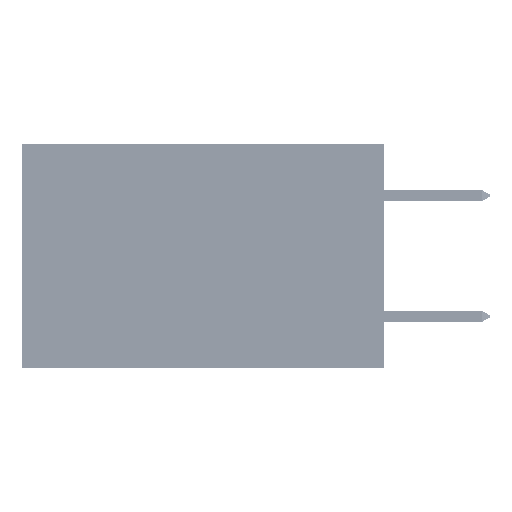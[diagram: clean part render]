
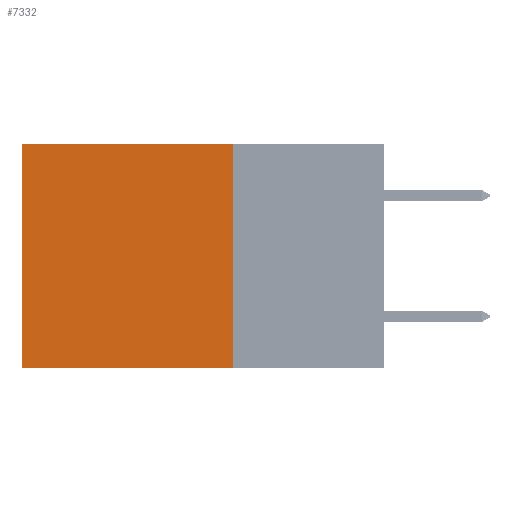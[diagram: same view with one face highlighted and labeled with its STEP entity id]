
A CAD part, left-side view. The second image highlights one B-rep face of the part: STEP entity #7332.
In plain terms, the highlighted planar face has unit normal (-1, 0, 0).
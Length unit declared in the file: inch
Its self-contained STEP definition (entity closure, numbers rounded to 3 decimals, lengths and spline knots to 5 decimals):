
#388 = CARTESIAN_POINT ( 'NONE',  ( 0.2875, 0.6, 0. ) ) ;
#1718 = DIRECTION ( 'NONE',  ( 0., 1., 0. ) ) ;
#2226 = DIRECTION ( 'NONE',  ( 1., 0., 0. ) ) ;
#3516 = AXIS2_PLACEMENT_3D ( 'NONE', #24717, #2226, #6004 ) ;
#3786 = VECTOR ( 'NONE', #7145, 39.37008 ) ;
#4323 = EDGE_LOOP ( 'NONE', ( #27714, #42991, #12882, #36826 ) ) ;
#5016 = EDGE_CURVE ( 'NONE', #23131, #36613, #47746, .T. ) ;
#6004 = DIRECTION ( 'NONE',  ( 0., 0., -1. ) ) ;
#6733 = CARTESIAN_POINT ( 'NONE',  ( 0.2875, 0.25, 0. ) ) ;
#7145 = DIRECTION ( 'NONE',  ( 0., 1., 0. ) ) ;
#7332 = ADVANCED_FACE ( 'NONE', ( #18770 ), #43321, .F. ) ;
#7511 = CARTESIAN_POINT ( 'NONE',  ( 0.2875, 0.6, 0. ) ) ;
#11528 = DIRECTION ( 'NONE',  ( 0., 0., -1. ) ) ;
#12882 = ORIENTED_EDGE ( 'NONE', *, *, #30175, .F. ) ;
#14334 = CARTESIAN_POINT ( 'NONE',  ( 0.2875, 0.6, -0.37 ) ) ;
#18770 = FACE_OUTER_BOUND ( 'NONE', #4323, .T. ) ;
#19137 = DIRECTION ( 'NONE',  ( 0., 0., -1. ) ) ;
#19555 = VERTEX_POINT ( 'NONE', #6733 ) ;
#21462 = VECTOR ( 'NONE', #11528, 39.37008 ) ;
#22094 = CARTESIAN_POINT ( 'NONE',  ( 0.2875, 0.25, 0. ) ) ;
#23131 = VERTEX_POINT ( 'NONE', #388 ) ;
#24717 = CARTESIAN_POINT ( 'NONE',  ( 0.2875, 0.25, 0. ) ) ;
#25836 = CARTESIAN_POINT ( 'NONE',  ( 0.2875, 0.25, -0.37 ) ) ;
#25905 = LINE ( 'NONE', #27673, #41194 ) ;
#27673 = CARTESIAN_POINT ( 'NONE',  ( 0.2875, 0.25, 0. ) ) ;
#27714 = ORIENTED_EDGE ( 'NONE', *, *, #5016, .T. ) ;
#27750 = EDGE_CURVE ( 'NONE', #19555, #23131, #25905, .T. ) ;
#28917 = VECTOR ( 'NONE', #19137, 39.37008 ) ;
#30101 = EDGE_CURVE ( 'NONE', #39556, #36613, #32620, .T. ) ;
#30175 = EDGE_CURVE ( 'NONE', #19555, #39556, #36176, .T. ) ;
#32620 = LINE ( 'NONE', #25836, #3786 ) ;
#36176 = LINE ( 'NONE', #22094, #21462 ) ;
#36613 = VERTEX_POINT ( 'NONE', #14334 ) ;
#36826 = ORIENTED_EDGE ( 'NONE', *, *, #27750, .T. ) ;
#39556 = VERTEX_POINT ( 'NONE', #45095 ) ;
#41194 = VECTOR ( 'NONE', #1718, 39.37008 ) ;
#42991 = ORIENTED_EDGE ( 'NONE', *, *, #30101, .F. ) ;
#43321 = PLANE ( 'NONE',  #3516 ) ;
#45095 = CARTESIAN_POINT ( 'NONE',  ( 0.2875, 0.25, -0.37 ) ) ;
#47746 = LINE ( 'NONE', #7511, #28917 ) ;
